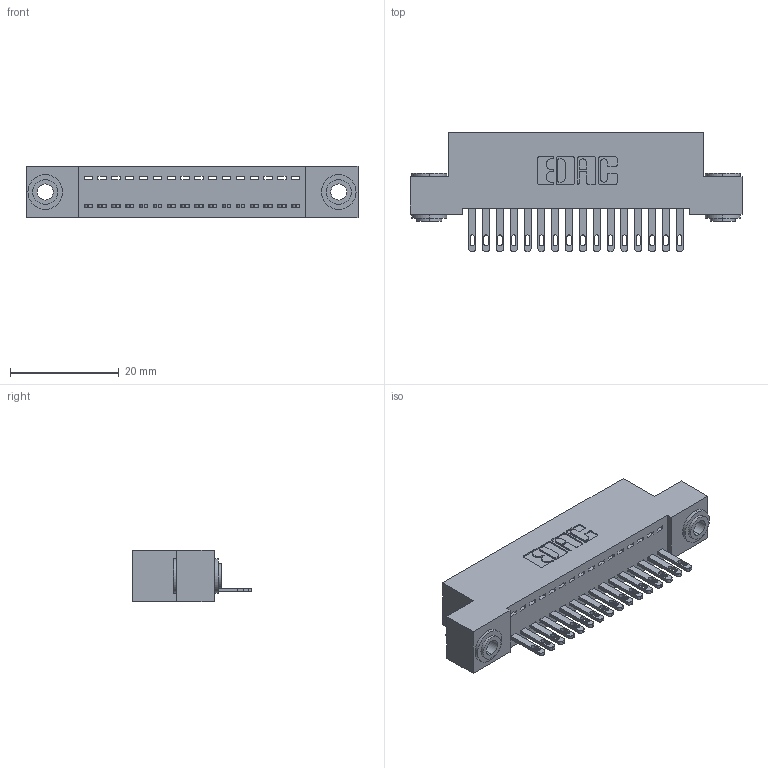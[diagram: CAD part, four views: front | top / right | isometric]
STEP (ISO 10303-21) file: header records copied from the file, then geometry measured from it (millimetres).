
FILE_DESCRIPTION (( 'STEP AP203' ), '1' );
FILE_NAME ('892-016-500-103.STEP', '2020-09-21T13:25:39', ( '' ), ( '' ), 'SwSTEP 2.0', 'SolidWorks 2020', '' );
FILE_SCHEMA (( 'CONFIG_CONTROL_DESIGN' ));
Length unit declared in the file: inch
Products named in the file (4): 342-250-002_345-250-002-102; 345-292-001_345-293-100; 842 Part_.156 TH; 892-016-500-103
Assembly tree (19 placements, depth 2):
  892-016-500-103
    842 Part_.156 TH
    345-292-001_345-293-100  x16
    342-250-002_345-250-002-102  x2
Bounding box: 60.96 x 21.85 x 9.4 mm (x, y, z)
Volume: 5281.9 mm3; surface area: 7528.5 mm2
Topology: 19 solids, 19 shells, 1012 faces, 3063 edges, 2038 vertices
Faces by surface type: plane 652, cylinder 352, cone 8
Entity records: 13592 total; most frequent: CARTESIAN_POINT 2325, ORIENTED_EDGE 2270, DIRECTION 2049, EDGE_CURVE 1135, LINE 979, VECTOR 979, VERTEX_POINT 754, AXIS2_PLACEMENT_3D 535
